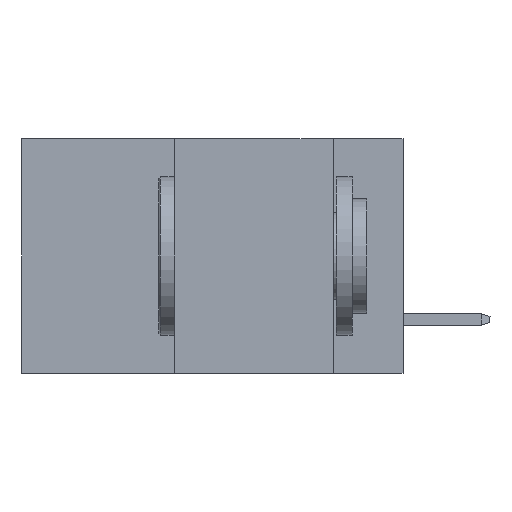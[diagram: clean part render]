
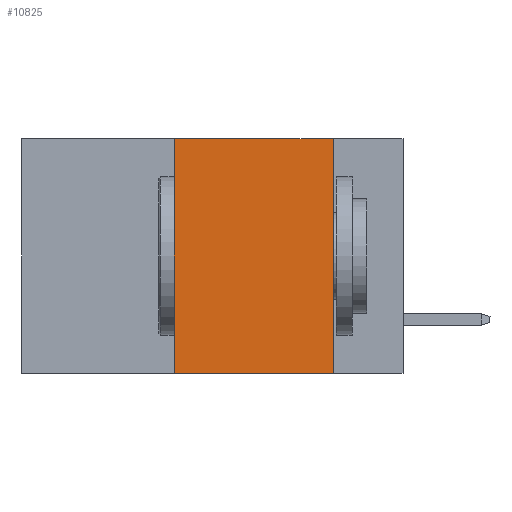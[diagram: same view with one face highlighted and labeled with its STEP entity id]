
A CAD part, left-side view. The second image highlights one B-rep face of the part: STEP entity #10825.
In plain terms, the highlighted planar face has unit normal (-1, 0, 0).
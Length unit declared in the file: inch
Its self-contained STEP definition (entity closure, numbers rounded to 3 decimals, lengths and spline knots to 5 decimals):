
#51 = CARTESIAN_POINT ( 'NONE',  ( 0., 0.36, 0. ) ) ;
#657 = VECTOR ( 'NONE', #2119, 39.37008 ) ;
#1060 = DIRECTION ( 'NONE',  ( 0., 0., -1. ) ) ;
#1320 = CARTESIAN_POINT ( 'NONE',  ( 0., 0.11, -0.37 ) ) ;
#1844 = ORIENTED_EDGE ( 'NONE', *, *, #9249, .F. ) ;
#1994 = FACE_OUTER_BOUND ( 'NONE', #10324, .T. ) ;
#2119 = DIRECTION ( 'NONE',  ( 0., 0., -1. ) ) ;
#2230 = CARTESIAN_POINT ( 'NONE',  ( 0., 0.11, 0. ) ) ;
#2486 = VECTOR ( 'NONE', #6505, 39.37008 ) ;
#3596 = DIRECTION ( 'NONE',  ( 0., 0., 1. ) ) ;
#3725 = VECTOR ( 'NONE', #3596, 39.37008 ) ;
#3905 = VERTEX_POINT ( 'NONE', #8549 ) ;
#4509 = LINE ( 'NONE', #51, #3725 ) ;
#4855 = EDGE_CURVE ( 'NONE', #6233, #9018, #4509, .T. ) ;
#4942 = VERTEX_POINT ( 'NONE', #1320 ) ;
#5164 = CARTESIAN_POINT ( 'NONE',  ( 0., 0.36, -0.37 ) ) ;
#5298 = DIRECTION ( 'NONE',  ( 0., -1., 0. ) ) ;
#5344 = PLANE ( 'NONE',  #8480 ) ;
#5463 = DIRECTION ( 'NONE',  ( 1., 0., 0. ) ) ;
#5496 = VECTOR ( 'NONE', #5298, 39.37008 ) ;
#6196 = CARTESIAN_POINT ( 'NONE',  ( 0., 0.6, 0. ) ) ;
#6233 = VERTEX_POINT ( 'NONE', #5164 ) ;
#6505 = DIRECTION ( 'NONE',  ( 0., -1., 0. ) ) ;
#6758 = EDGE_CURVE ( 'NONE', #9018, #3905, #10936, .T. ) ;
#7033 = CARTESIAN_POINT ( 'NONE',  ( 0., 0.36, 0. ) ) ;
#7224 = ORIENTED_EDGE ( 'NONE', *, *, #6758, .F. ) ;
#8316 = CARTESIAN_POINT ( 'NONE',  ( 0., 0.6, 0. ) ) ;
#8480 = AXIS2_PLACEMENT_3D ( 'NONE', #6196, #5463, #1060 ) ;
#8549 = CARTESIAN_POINT ( 'NONE',  ( 0., 0.11, 0. ) ) ;
#8726 = CARTESIAN_POINT ( 'NONE',  ( 0., 0.6, -0.37 ) ) ;
#8977 = EDGE_CURVE ( 'NONE', #6233, #4942, #10469, .T. ) ;
#9018 = VERTEX_POINT ( 'NONE', #7033 ) ;
#9249 = EDGE_CURVE ( 'NONE', #3905, #4942, #10172, .T. ) ;
#10149 = ORIENTED_EDGE ( 'NONE', *, *, #8977, .T. ) ;
#10172 = LINE ( 'NONE', #2230, #657 ) ;
#10324 = EDGE_LOOP ( 'NONE', ( #1844, #7224, #10493, #10149 ) ) ;
#10469 = LINE ( 'NONE', #8726, #5496 ) ;
#10493 = ORIENTED_EDGE ( 'NONE', *, *, #4855, .F. ) ;
#10825 = ADVANCED_FACE ( 'NONE', ( #1994 ), #5344, .F. ) ;
#10936 = LINE ( 'NONE', #8316, #2486 ) ;
